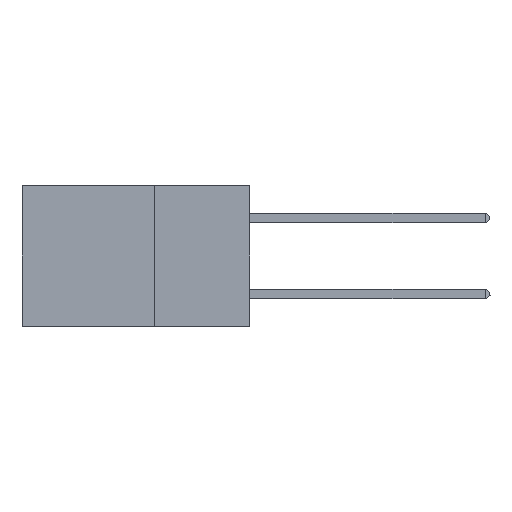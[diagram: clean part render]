
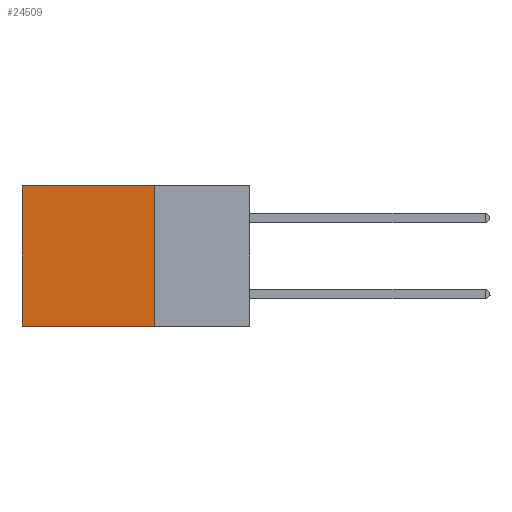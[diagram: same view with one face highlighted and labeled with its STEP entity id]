
A CAD part, left-side view. The second image highlights one B-rep face of the part: STEP entity #24509.
In plain terms, the highlighted planar face has unit normal (-1, 0, 0).
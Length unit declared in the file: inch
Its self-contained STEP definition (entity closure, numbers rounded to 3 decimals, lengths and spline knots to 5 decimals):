
#1014 = VECTOR ( 'NONE', #25473, 39.37008 ) ;
#2050 = DIRECTION ( 'NONE',  ( 0., 1., 0. ) ) ;
#2689 = LINE ( 'NONE', #8540, #26401 ) ;
#3104 = LINE ( 'NONE', #18850, #25091 ) ;
#4886 = EDGE_CURVE ( 'NONE', #6109, #9193, #2689, .T. ) ;
#5467 = CARTESIAN_POINT ( 'NONE',  ( 0.2875, 0.6, 0. ) ) ;
#6109 = VERTEX_POINT ( 'NONE', #30706 ) ;
#8540 = CARTESIAN_POINT ( 'NONE',  ( 0.2875, 0.25, 0. ) ) ;
#9193 = VERTEX_POINT ( 'NONE', #16363 ) ;
#10447 = FACE_OUTER_BOUND ( 'NONE', #25722, .T. ) ;
#10658 = DIRECTION ( 'NONE',  ( 1., 0., 0. ) ) ;
#13023 = VERTEX_POINT ( 'NONE', #42135 ) ;
#16363 = CARTESIAN_POINT ( 'NONE',  ( 0.2875, 0.6, 0. ) ) ;
#18850 = CARTESIAN_POINT ( 'NONE',  ( 0.2875, 0.25, 0. ) ) ;
#21579 = VECTOR ( 'NONE', #2050, 39.37008 ) ;
#24509 = ADVANCED_FACE ( 'NONE', ( #10447 ), #27006, .F. ) ;
#25091 = VECTOR ( 'NONE', #28519, 39.37008 ) ;
#25354 = ORIENTED_EDGE ( 'NONE', *, *, #25884, .T. ) ;
#25473 = DIRECTION ( 'NONE',  ( 0., 0., -1. ) ) ;
#25722 = EDGE_LOOP ( 'NONE', ( #25354, #30573, #40664, #36978 ) ) ;
#25884 = EDGE_CURVE ( 'NONE', #9193, #27567, #41415, .T. ) ;
#26401 = VECTOR ( 'NONE', #42085, 39.37008 ) ;
#26792 = CARTESIAN_POINT ( 'NONE',  ( 0.2875, 0.25, 0. ) ) ;
#27006 = PLANE ( 'NONE',  #29125 ) ;
#27567 = VERTEX_POINT ( 'NONE', #33880 ) ;
#28519 = DIRECTION ( 'NONE',  ( 0., 0., -1. ) ) ;
#29125 = AXIS2_PLACEMENT_3D ( 'NONE', #26792, #10658, #29591 ) ;
#29591 = DIRECTION ( 'NONE',  ( 0., 0., -1. ) ) ;
#30573 = ORIENTED_EDGE ( 'NONE', *, *, #38418, .F. ) ;
#30706 = CARTESIAN_POINT ( 'NONE',  ( 0.2875, 0.25, 0. ) ) ;
#31112 = CARTESIAN_POINT ( 'NONE',  ( 0.2875, 0.25, -0.37 ) ) ;
#33880 = CARTESIAN_POINT ( 'NONE',  ( 0.2875, 0.6, -0.37 ) ) ;
#36978 = ORIENTED_EDGE ( 'NONE', *, *, #4886, .T. ) ;
#37990 = LINE ( 'NONE', #31112, #21579 ) ;
#38418 = EDGE_CURVE ( 'NONE', #13023, #27567, #37990, .T. ) ;
#39796 = EDGE_CURVE ( 'NONE', #6109, #13023, #3104, .T. ) ;
#40664 = ORIENTED_EDGE ( 'NONE', *, *, #39796, .F. ) ;
#41415 = LINE ( 'NONE', #5467, #1014 ) ;
#42085 = DIRECTION ( 'NONE',  ( 0., 1., 0. ) ) ;
#42135 = CARTESIAN_POINT ( 'NONE',  ( 0.2875, 0.25, -0.37 ) ) ;
